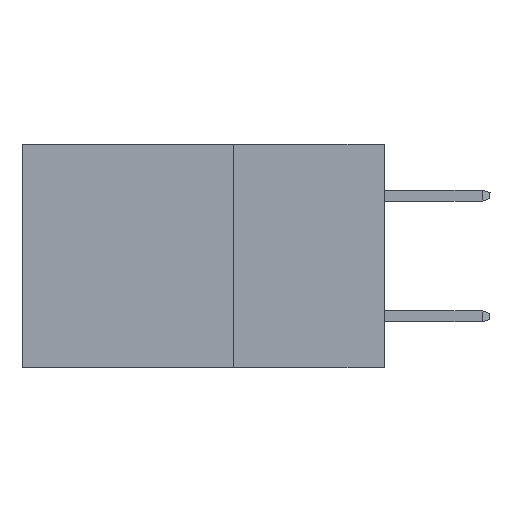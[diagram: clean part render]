
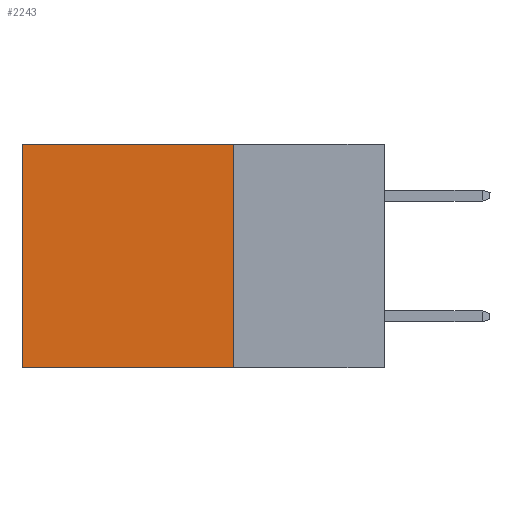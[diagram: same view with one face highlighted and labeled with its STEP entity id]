
A CAD part, left-side view. The second image highlights one B-rep face of the part: STEP entity #2243.
In plain terms, the highlighted planar face has unit normal (-1, 0, 0).
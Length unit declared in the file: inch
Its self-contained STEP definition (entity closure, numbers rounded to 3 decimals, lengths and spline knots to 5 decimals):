
#91 = EDGE_CURVE ( 'NONE', #6775, #2127, #21710, .T. ) ;
#552 = VECTOR ( 'NONE', #3554, 39.37008 ) ;
#2124 = DIRECTION ( 'NONE',  ( 0., 0., -1. ) ) ;
#2127 = VERTEX_POINT ( 'NONE', #31928 ) ;
#2243 = ADVANCED_FACE ( 'NONE', ( #31955 ), #4032, .F. ) ;
#3554 = DIRECTION ( 'NONE',  ( 0., 1., 0. ) ) ;
#3683 = CARTESIAN_POINT ( 'NONE',  ( 0.298, 0.25, 0. ) ) ;
#4032 = PLANE ( 'NONE',  #17546 ) ;
#6404 = VECTOR ( 'NONE', #2124, 39.37008 ) ;
#6613 = DIRECTION ( 'NONE',  ( 0., 0., -1. ) ) ;
#6775 = VERTEX_POINT ( 'NONE', #19852 ) ;
#9238 = EDGE_LOOP ( 'NONE', ( #24296, #29491, #26909, #19485 ) ) ;
#10019 = LINE ( 'NONE', #30364, #6404 ) ;
#12312 = VERTEX_POINT ( 'NONE', #31059 ) ;
#14858 = VECTOR ( 'NONE', #22045, 39.37008 ) ;
#15690 = LINE ( 'NONE', #29545, #14858 ) ;
#17546 = AXIS2_PLACEMENT_3D ( 'NONE', #24322, #22092, #6613 ) ;
#18469 = VERTEX_POINT ( 'NONE', #23785 ) ;
#19485 = ORIENTED_EDGE ( 'NONE', *, *, #91, .T. ) ;
#19852 = CARTESIAN_POINT ( 'NONE',  ( 0.298, 0.25, 0. ) ) ;
#20665 = EDGE_CURVE ( 'NONE', #2127, #12312, #10019, .T. ) ;
#21042 = EDGE_CURVE ( 'NONE', #6775, #18469, #15690, .T. ) ;
#21614 = LINE ( 'NONE', #33287, #552 ) ;
#21710 = LINE ( 'NONE', #3683, #29718 ) ;
#21730 = DIRECTION ( 'NONE',  ( 0., 1., 0. ) ) ;
#22045 = DIRECTION ( 'NONE',  ( 0., 0., -1. ) ) ;
#22092 = DIRECTION ( 'NONE',  ( 1., 0., 0. ) ) ;
#22261 = EDGE_CURVE ( 'NONE', #18469, #12312, #21614, .T. ) ;
#23785 = CARTESIAN_POINT ( 'NONE',  ( 0.298, 0.25, -0.37 ) ) ;
#24296 = ORIENTED_EDGE ( 'NONE', *, *, #20665, .T. ) ;
#24322 = CARTESIAN_POINT ( 'NONE',  ( 0.298, 0.25, 0. ) ) ;
#26909 = ORIENTED_EDGE ( 'NONE', *, *, #21042, .F. ) ;
#29491 = ORIENTED_EDGE ( 'NONE', *, *, #22261, .F. ) ;
#29545 = CARTESIAN_POINT ( 'NONE',  ( 0.298, 0.25, 0. ) ) ;
#29718 = VECTOR ( 'NONE', #21730, 39.37008 ) ;
#30364 = CARTESIAN_POINT ( 'NONE',  ( 0.298, 0.6, 0. ) ) ;
#31059 = CARTESIAN_POINT ( 'NONE',  ( 0.298, 0.6, -0.37 ) ) ;
#31928 = CARTESIAN_POINT ( 'NONE',  ( 0.298, 0.6, 0. ) ) ;
#31955 = FACE_OUTER_BOUND ( 'NONE', #9238, .T. ) ;
#33287 = CARTESIAN_POINT ( 'NONE',  ( 0.298, 0.25, -0.37 ) ) ;
